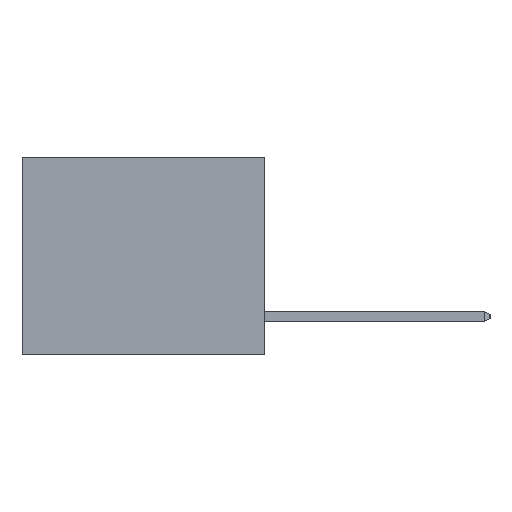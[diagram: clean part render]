
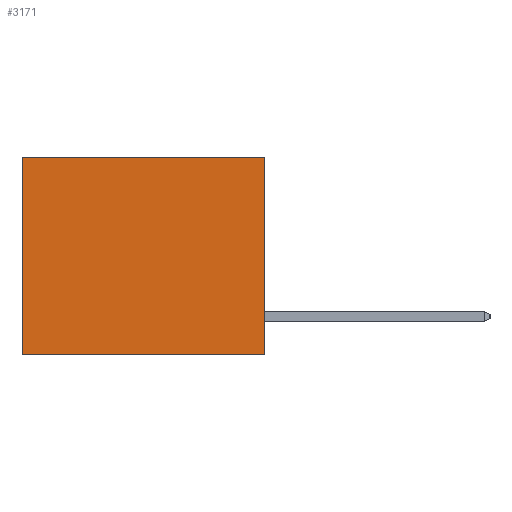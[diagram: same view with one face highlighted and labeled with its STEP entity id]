
A CAD part, left-side view. The second image highlights one B-rep face of the part: STEP entity #3171.
In plain terms, the highlighted planar face has unit normal (-1, 0, 0).
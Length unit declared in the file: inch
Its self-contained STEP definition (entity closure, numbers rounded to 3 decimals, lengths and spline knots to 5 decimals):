
#60 = VERTEX_POINT ( 'NONE', #18274 ) ;
#62 = VECTOR ( 'NONE', #13792, 39.37008 ) ;
#271 = CARTESIAN_POINT ( 'NONE',  ( 0.3165, 0.6, -0.49 ) ) ;
#384 = ORIENTED_EDGE ( 'NONE', *, *, #1472, .F. ) ;
#509 = DIRECTION ( 'NONE',  ( 0., 1., 0. ) ) ;
#1133 = LINE ( 'NONE', #18820, #62 ) ;
#1330 = CARTESIAN_POINT ( 'NONE',  ( 0.3165, 0., -0.49 ) ) ;
#1472 = EDGE_CURVE ( 'NONE', #19502, #11356, #1133, .T. ) ;
#1890 = DIRECTION ( 'NONE',  ( 0., 0., -1. ) ) ;
#1967 = LINE ( 'NONE', #3662, #19571 ) ;
#2142 = CARTESIAN_POINT ( 'NONE',  ( 0.3165, 0., 0. ) ) ;
#2319 = LINE ( 'NONE', #2142, #10316 ) ;
#2486 = CARTESIAN_POINT ( 'NONE',  ( 0.3165, 0., 0. ) ) ;
#2573 = ORIENTED_EDGE ( 'NONE', *, *, #13518, .T. ) ;
#3026 = DIRECTION ( 'NONE',  ( 0., 0., -1. ) ) ;
#3171 = ADVANCED_FACE ( 'NONE', ( #19463 ), #16519, .F. ) ;
#3433 = DIRECTION ( 'NONE',  ( 0., 1., 0. ) ) ;
#3662 = CARTESIAN_POINT ( 'NONE',  ( 0.3165, 0., -0.49 ) ) ;
#5955 = EDGE_CURVE ( 'NONE', #60, #15644, #19330, .T. ) ;
#7003 = AXIS2_PLACEMENT_3D ( 'NONE', #1330, #16661, #3026 ) ;
#10316 = VECTOR ( 'NONE', #509, 39.37008 ) ;
#11356 = VERTEX_POINT ( 'NONE', #16242 ) ;
#13518 = EDGE_CURVE ( 'NONE', #19502, #60, #2319, .T. ) ;
#13792 = DIRECTION ( 'NONE',  ( 0., 0., -1. ) ) ;
#14237 = ORIENTED_EDGE ( 'NONE', *, *, #5955, .T. ) ;
#14757 = EDGE_LOOP ( 'NONE', ( #14237, #14808, #384, #2573 ) ) ;
#14808 = ORIENTED_EDGE ( 'NONE', *, *, #19985, .F. ) ;
#15644 = VERTEX_POINT ( 'NONE', #18152 ) ;
#16242 = CARTESIAN_POINT ( 'NONE',  ( 0.3165, 0., -0.49 ) ) ;
#16519 = PLANE ( 'NONE',  #7003 ) ;
#16661 = DIRECTION ( 'NONE',  ( 1., 0., 0. ) ) ;
#18152 = CARTESIAN_POINT ( 'NONE',  ( 0.3165, 0.6, -0.49 ) ) ;
#18274 = CARTESIAN_POINT ( 'NONE',  ( 0.3165, 0.6, 0. ) ) ;
#18787 = VECTOR ( 'NONE', #1890, 39.37008 ) ;
#18820 = CARTESIAN_POINT ( 'NONE',  ( 0.3165, 0., -0.49 ) ) ;
#19330 = LINE ( 'NONE', #271, #18787 ) ;
#19463 = FACE_OUTER_BOUND ( 'NONE', #14757, .T. ) ;
#19502 = VERTEX_POINT ( 'NONE', #2486 ) ;
#19571 = VECTOR ( 'NONE', #3433, 39.37008 ) ;
#19985 = EDGE_CURVE ( 'NONE', #11356, #15644, #1967, .T. ) ;
